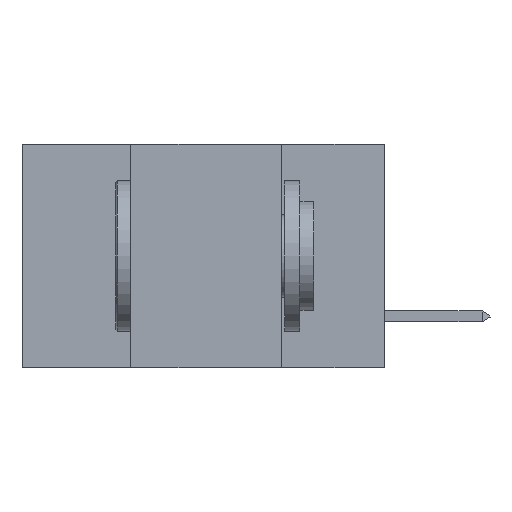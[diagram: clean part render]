
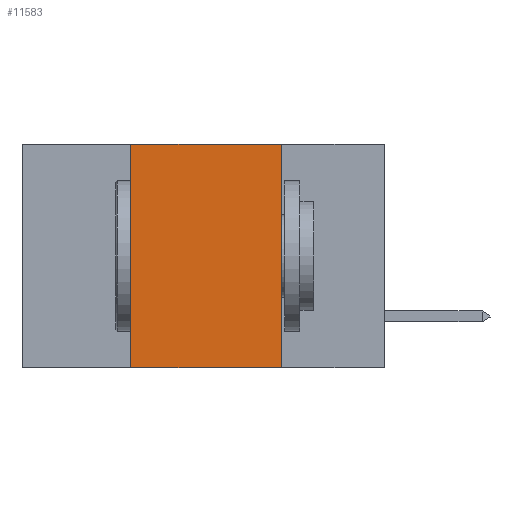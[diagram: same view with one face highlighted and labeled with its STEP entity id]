
A CAD part, left-side view. The second image highlights one B-rep face of the part: STEP entity #11583.
In plain terms, the highlighted planar face has unit normal (-1, 0, 0).
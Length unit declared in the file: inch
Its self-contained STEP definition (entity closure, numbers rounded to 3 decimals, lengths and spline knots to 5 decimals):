
#1090 = LINE ( 'NONE', #7375, #4242 ) ;
#1172 = LINE ( 'NONE', #2299, #16361 ) ;
#1257 = VERTEX_POINT ( 'NONE', #4583 ) ;
#1271 = PLANE ( 'NONE',  #12670 ) ;
#1625 = ORIENTED_EDGE ( 'NONE', *, *, #10679, .F. ) ;
#2299 = CARTESIAN_POINT ( 'NONE',  ( 0., 0.42, 0. ) ) ;
#2518 = VERTEX_POINT ( 'NONE', #9617 ) ;
#2603 = ORIENTED_EDGE ( 'NONE', *, *, #14769, .F. ) ;
#2828 = DIRECTION ( 'NONE',  ( 0., 0., -1. ) ) ;
#3745 = VERTEX_POINT ( 'NONE', #5836 ) ;
#4242 = VECTOR ( 'NONE', #18634, 39.37008 ) ;
#4257 = LINE ( 'NONE', #14592, #18616 ) ;
#4365 = DIRECTION ( 'NONE',  ( 0., 0., -1. ) ) ;
#4489 = CARTESIAN_POINT ( 'NONE',  ( 0., 0.42, -0.37 ) ) ;
#4583 = CARTESIAN_POINT ( 'NONE',  ( 0., 0.42, 0. ) ) ;
#5245 = ORIENTED_EDGE ( 'NONE', *, *, #18658, .F. ) ;
#5311 = DIRECTION ( 'NONE',  ( 0., -1., 0. ) ) ;
#5836 = CARTESIAN_POINT ( 'NONE',  ( 0., 0.17, 0. ) ) ;
#5873 = FACE_OUTER_BOUND ( 'NONE', #10275, .T. ) ;
#7375 = CARTESIAN_POINT ( 'NONE',  ( 0., 0.6, 0. ) ) ;
#9617 = CARTESIAN_POINT ( 'NONE',  ( 0., 0.17, -0.37 ) ) ;
#10126 = VERTEX_POINT ( 'NONE', #4489 ) ;
#10275 = EDGE_LOOP ( 'NONE', ( #5245, #1625, #2603, #14817 ) ) ;
#10679 = EDGE_CURVE ( 'NONE', #1257, #3745, #1090, .T. ) ;
#10835 = VECTOR ( 'NONE', #5311, 39.37008 ) ;
#11583 = ADVANCED_FACE ( 'NONE', ( #5873 ), #1271, .F. ) ;
#11749 = DIRECTION ( 'NONE',  ( 1., 0., 0. ) ) ;
#12670 = AXIS2_PLACEMENT_3D ( 'NONE', #17336, #11749, #2828 ) ;
#14055 = CARTESIAN_POINT ( 'NONE',  ( 0., 0.6, -0.37 ) ) ;
#14168 = LINE ( 'NONE', #14055, #10835 ) ;
#14592 = CARTESIAN_POINT ( 'NONE',  ( 0., 0.17, 0. ) ) ;
#14769 = EDGE_CURVE ( 'NONE', #10126, #1257, #1172, .T. ) ;
#14817 = ORIENTED_EDGE ( 'NONE', *, *, #15345, .T. ) ;
#15345 = EDGE_CURVE ( 'NONE', #10126, #2518, #14168, .T. ) ;
#16361 = VECTOR ( 'NONE', #18262, 39.37008 ) ;
#17336 = CARTESIAN_POINT ( 'NONE',  ( 0., 0.6, 0. ) ) ;
#18262 = DIRECTION ( 'NONE',  ( 0., 0., 1. ) ) ;
#18616 = VECTOR ( 'NONE', #4365, 39.37008 ) ;
#18634 = DIRECTION ( 'NONE',  ( 0., -1., 0. ) ) ;
#18658 = EDGE_CURVE ( 'NONE', #3745, #2518, #4257, .T. ) ;
